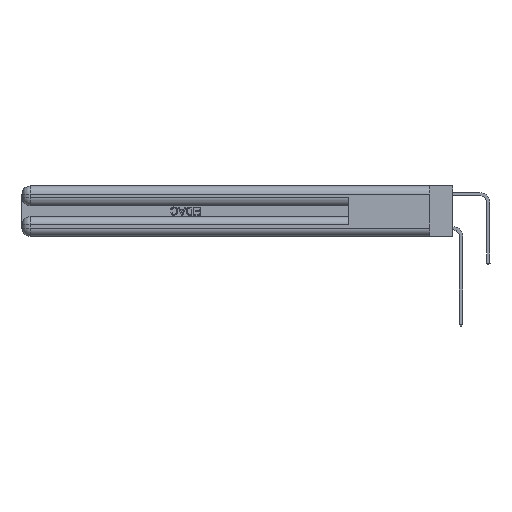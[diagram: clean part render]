
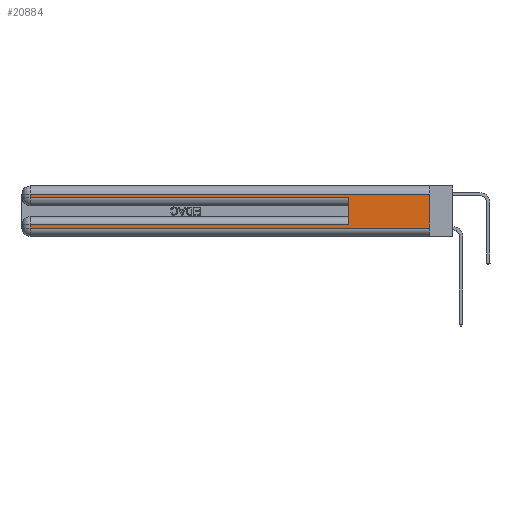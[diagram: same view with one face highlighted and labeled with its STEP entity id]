
A CAD part, left-side view. The second image highlights one B-rep face of the part: STEP entity #20884.
In plain terms, the highlighted planar face has unit normal (-1, 0, 0).
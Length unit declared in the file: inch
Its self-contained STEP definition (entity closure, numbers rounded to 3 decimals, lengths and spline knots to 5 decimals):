
#2243 = CARTESIAN_POINT ( 'NONE',  ( 0., 2.94, 0.37 ) ) ;
#2603 = VECTOR ( 'NONE', #30470, 39.37008 ) ;
#3063 = VERTEX_POINT ( 'NONE', #20276 ) ;
#3753 = DIRECTION ( 'NONE',  ( 0., -1., 0. ) ) ;
#4077 = CARTESIAN_POINT ( 'NONE',  ( 0., 2.94, 0.06 ) ) ;
#4106 = CARTESIAN_POINT ( 'NONE',  ( 0., 2.94, 0.085 ) ) ;
#4277 = PLANE ( 'NONE',  #4902 ) ;
#4735 = LINE ( 'NONE', #15204, #21043 ) ;
#4788 = VECTOR ( 'NONE', #22826, 39.37008 ) ;
#4902 = AXIS2_PLACEMENT_3D ( 'NONE', #11491, #29563, #11617 ) ;
#6604 = CARTESIAN_POINT ( 'NONE',  ( 0., 0., 0.085 ) ) ;
#7250 = VECTOR ( 'NONE', #26029, 39.37008 ) ;
#7707 = VERTEX_POINT ( 'NONE', #23299 ) ;
#8349 = ORIENTED_EDGE ( 'NONE', *, *, #21856, .T. ) ;
#9508 = EDGE_CURVE ( 'NONE', #10052, #22985, #23479, .T. ) ;
#10052 = VERTEX_POINT ( 'NONE', #20458 ) ;
#10337 = ORIENTED_EDGE ( 'NONE', *, *, #32990, .T. ) ;
#10714 = VERTEX_POINT ( 'NONE', #4106 ) ;
#10877 = LINE ( 'NONE', #6604, #16389 ) ;
#11491 = CARTESIAN_POINT ( 'NONE',  ( 0., 0., 0.37 ) ) ;
#11617 = DIRECTION ( 'NONE',  ( 0., 0., -1. ) ) ;
#12423 = ORIENTED_EDGE ( 'NONE', *, *, #22230, .F. ) ;
#13352 = ORIENTED_EDGE ( 'NONE', *, *, #22960, .T. ) ;
#14101 = VERTEX_POINT ( 'NONE', #17989 ) ;
#14912 = VECTOR ( 'NONE', #22983, 39.37008 ) ;
#15204 = CARTESIAN_POINT ( 'NONE',  ( 0., 2.94, 0.37 ) ) ;
#15270 = CARTESIAN_POINT ( 'NONE',  ( 0., 0.6, 0.145 ) ) ;
#16389 = VECTOR ( 'NONE', #22136, 39.37008 ) ;
#17630 = ORIENTED_EDGE ( 'NONE', *, *, #26644, .T. ) ;
#17791 = CARTESIAN_POINT ( 'NONE',  ( 0., 0., 0.31 ) ) ;
#17989 = CARTESIAN_POINT ( 'NONE',  ( 0., 0.6, 0.085 ) ) ;
#18062 = EDGE_LOOP ( 'NONE', ( #12423, #23577, #17630, #8349, #18108, #10337, #13352, #19323 ) ) ;
#18108 = ORIENTED_EDGE ( 'NONE', *, *, #30771, .F. ) ;
#18445 = CARTESIAN_POINT ( 'NONE',  ( 0., 0., 0.285 ) ) ;
#18862 = LINE ( 'NONE', #2243, #20083 ) ;
#19323 = ORIENTED_EDGE ( 'NONE', *, *, #32361, .T. ) ;
#20083 = VECTOR ( 'NONE', #23156, 39.37008 ) ;
#20276 = CARTESIAN_POINT ( 'NONE',  ( 0., 0., 0.06 ) ) ;
#20458 = CARTESIAN_POINT ( 'NONE',  ( 0., 0., 0.31 ) ) ;
#20884 = ADVANCED_FACE ( 'NONE', ( #21939 ), #4277, .F. ) ;
#21043 = VECTOR ( 'NONE', #22583, 39.37008 ) ;
#21856 = EDGE_CURVE ( 'NONE', #25858, #7707, #25585, .T. ) ;
#21939 = FACE_OUTER_BOUND ( 'NONE', #18062, .T. ) ;
#22136 = DIRECTION ( 'NONE',  ( 0., 1., 0. ) ) ;
#22230 = EDGE_CURVE ( 'NONE', #10052, #3063, #32475, .T. ) ;
#22583 = DIRECTION ( 'NONE',  ( 0., 0., -1. ) ) ;
#22826 = DIRECTION ( 'NONE',  ( 0., 1., 0. ) ) ;
#22873 = CARTESIAN_POINT ( 'NONE',  ( 0., 0., 0.37 ) ) ;
#22960 = EDGE_CURVE ( 'NONE', #10714, #31285, #18862, .T. ) ;
#22983 = DIRECTION ( 'NONE',  ( 0., 0., -1. ) ) ;
#22985 = VERTEX_POINT ( 'NONE', #25726 ) ;
#23156 = DIRECTION ( 'NONE',  ( 0., 0., -1. ) ) ;
#23299 = CARTESIAN_POINT ( 'NONE',  ( 0., 0.6, 0.285 ) ) ;
#23479 = LINE ( 'NONE', #17791, #4788 ) ;
#23577 = ORIENTED_EDGE ( 'NONE', *, *, #9508, .T. ) ;
#24041 = CARTESIAN_POINT ( 'NONE',  ( 0., 2.94, 0.285 ) ) ;
#25269 = VECTOR ( 'NONE', #3753, 39.37008 ) ;
#25585 = LINE ( 'NONE', #18445, #7250 ) ;
#25726 = CARTESIAN_POINT ( 'NONE',  ( 0., 2.94, 0.31 ) ) ;
#25858 = VERTEX_POINT ( 'NONE', #24041 ) ;
#26029 = DIRECTION ( 'NONE',  ( 0., -1., 0. ) ) ;
#26597 = CARTESIAN_POINT ( 'NONE',  ( 0., 0., 0.06 ) ) ;
#26644 = EDGE_CURVE ( 'NONE', #22985, #25858, #4735, .T. ) ;
#26856 = LINE ( 'NONE', #26597, #25269 ) ;
#29563 = DIRECTION ( 'NONE',  ( 1., 0., 0. ) ) ;
#30470 = DIRECTION ( 'NONE',  ( 0., 0., 1. ) ) ;
#30771 = EDGE_CURVE ( 'NONE', #14101, #7707, #31706, .T. ) ;
#31285 = VERTEX_POINT ( 'NONE', #4077 ) ;
#31706 = LINE ( 'NONE', #15270, #2603 ) ;
#32361 = EDGE_CURVE ( 'NONE', #31285, #3063, #26856, .T. ) ;
#32475 = LINE ( 'NONE', #22873, #14912 ) ;
#32990 = EDGE_CURVE ( 'NONE', #14101, #10714, #10877, .T. ) ;
